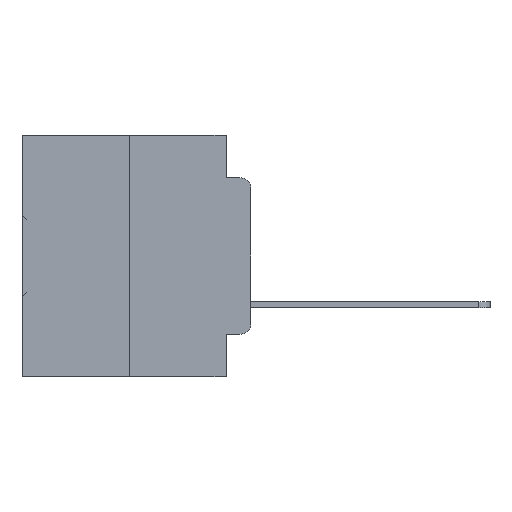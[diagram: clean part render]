
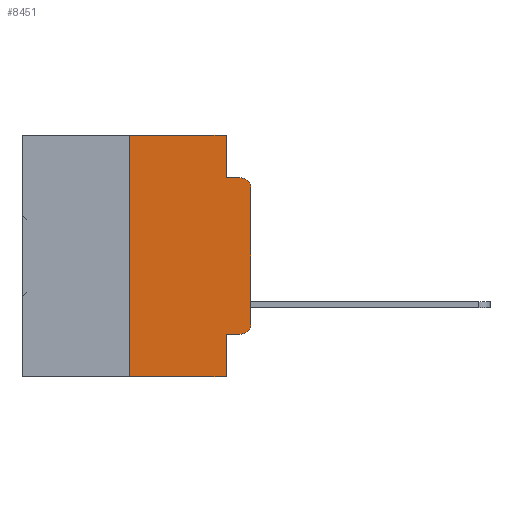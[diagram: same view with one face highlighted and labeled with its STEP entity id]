
A CAD part, left-side view. The second image highlights one B-rep face of the part: STEP entity #8451.
In plain terms, the highlighted planar face has unit normal (-1, 0, 0).
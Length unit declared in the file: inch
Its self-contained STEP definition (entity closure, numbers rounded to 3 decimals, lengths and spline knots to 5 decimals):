
#79 = EDGE_CURVE ( 'NONE', #17918, #13005, #28951, .T. ) ;
#101 = CARTESIAN_POINT ( 'NONE',  ( 0., 0.473, -0.5 ) ) ;
#487 = EDGE_CURVE ( 'NONE', #1792, #5767, #3883, .T. ) ;
#1195 = CARTESIAN_POINT ( 'NONE',  ( 0., 0.051, -0.4115 ) ) ;
#1426 = CIRCLE ( 'NONE', #29211, 0.02 ) ;
#1541 = VERTEX_POINT ( 'NONE', #7631 ) ;
#1792 = VERTEX_POINT ( 'NONE', #15027 ) ;
#2747 = EDGE_LOOP ( 'NONE', ( #7421, #23309, #15810, #28493, #32757, #30654, #3404, #32792, #27252, #3438 ) ) ;
#3170 = PLANE ( 'NONE',  #5697 ) ;
#3185 = EDGE_CURVE ( 'NONE', #1541, #13005, #27560, .T. ) ;
#3294 = DIRECTION ( 'NONE',  ( 0., 0., -1. ) ) ;
#3404 = ORIENTED_EDGE ( 'NONE', *, *, #3185, .T. ) ;
#3438 = ORIENTED_EDGE ( 'NONE', *, *, #20237, .T. ) ;
#3822 = VECTOR ( 'NONE', #32529, 39.37008 ) ;
#3883 = LINE ( 'NONE', #28431, #18070 ) ;
#4495 = CARTESIAN_POINT ( 'NONE',  ( 0., 0.051, 0. ) ) ;
#4998 = CARTESIAN_POINT ( 'NONE',  ( 0., 0., -0.1085 ) ) ;
#5225 = EDGE_CURVE ( 'NONE', #13765, #7297, #27836, .T. ) ;
#5697 = AXIS2_PLACEMENT_3D ( 'NONE', #14611, #20266, #3294 ) ;
#5767 = VERTEX_POINT ( 'NONE', #17756 ) ;
#5954 = DIRECTION ( 'NONE',  ( 0., -1., 0. ) ) ;
#7297 = VERTEX_POINT ( 'NONE', #11140 ) ;
#7421 = ORIENTED_EDGE ( 'NONE', *, *, #27356, .T. ) ;
#7631 = CARTESIAN_POINT ( 'NONE',  ( 0., 0.25, -0.5 ) ) ;
#8050 = LINE ( 'NONE', #35789, #15549 ) ;
#8303 = DIRECTION ( 'NONE',  ( 0., 0., 1. ) ) ;
#8451 = ADVANCED_FACE ( 'NONE', ( #18444 ), #3170, .F. ) ;
#9297 = DIRECTION ( 'NONE',  ( 0., -1., 0. ) ) ;
#11140 = CARTESIAN_POINT ( 'NONE',  ( 0., 0.02, -0.0885 ) ) ;
#11480 = LINE ( 'NONE', #25296, #18086 ) ;
#12324 = VECTOR ( 'NONE', #32002, 39.37008 ) ;
#12492 = DIRECTION ( 'NONE',  ( -1., 0., 0. ) ) ;
#13005 = VERTEX_POINT ( 'NONE', #32638 ) ;
#13181 = LINE ( 'NONE', #4495, #3822 ) ;
#13234 = CARTESIAN_POINT ( 'NONE',  ( 0., 0.02, -0.3915 ) ) ;
#13443 = AXIS2_PLACEMENT_3D ( 'NONE', #29235, #12492, #31969 ) ;
#13765 = VERTEX_POINT ( 'NONE', #4998 ) ;
#14611 = CARTESIAN_POINT ( 'NONE',  ( 0., 0.473, 0. ) ) ;
#15027 = CARTESIAN_POINT ( 'NONE',  ( 0., 0.25, 0. ) ) ;
#15381 = CARTESIAN_POINT ( 'NONE',  ( 0., 0.051, 0. ) ) ;
#15549 = VECTOR ( 'NONE', #35906, 39.37008 ) ;
#15810 = ORIENTED_EDGE ( 'NONE', *, *, #26135, .F. ) ;
#15893 = VECTOR ( 'NONE', #29018, 39.37008 ) ;
#16059 = DIRECTION ( 'NONE',  ( 0., 0., -1. ) ) ;
#17756 = CARTESIAN_POINT ( 'NONE',  ( 0., 0.051, 0. ) ) ;
#17918 = VERTEX_POINT ( 'NONE', #1195 ) ;
#18070 = VECTOR ( 'NONE', #5954, 39.37008 ) ;
#18086 = VECTOR ( 'NONE', #8303, 39.37008 ) ;
#18444 = FACE_OUTER_BOUND ( 'NONE', #2747, .T. ) ;
#19064 = EDGE_CURVE ( 'NONE', #17918, #32541, #35606, .T. ) ;
#19579 = CARTESIAN_POINT ( 'NONE',  ( 0., 0.051, -0.0885 ) ) ;
#20128 = VECTOR ( 'NONE', #30985, 39.37008 ) ;
#20237 = EDGE_CURVE ( 'NONE', #32541, #23037, #1426, .T. ) ;
#20266 = DIRECTION ( 'NONE',  ( 1., 0., 0. ) ) ;
#23037 = VERTEX_POINT ( 'NONE', #29609 ) ;
#23309 = ORIENTED_EDGE ( 'NONE', *, *, #5225, .T. ) ;
#23374 = LINE ( 'NONE', #26274, #15893 ) ;
#24098 = CARTESIAN_POINT ( 'NONE',  ( 0., 0.02, -0.4115 ) ) ;
#25296 = CARTESIAN_POINT ( 'NONE',  ( 0., 0., 0. ) ) ;
#26135 = EDGE_CURVE ( 'NONE', #32149, #7297, #8050, .T. ) ;
#26274 = CARTESIAN_POINT ( 'NONE',  ( 0., 0.25, 0. ) ) ;
#27252 = ORIENTED_EDGE ( 'NONE', *, *, #19064, .T. ) ;
#27356 = EDGE_CURVE ( 'NONE', #23037, #13765, #11480, .T. ) ;
#27521 = VECTOR ( 'NONE', #9297, 39.37008 ) ;
#27560 = LINE ( 'NONE', #101, #20128 ) ;
#27836 = CIRCLE ( 'NONE', #13443, 0.02 ) ;
#28431 = CARTESIAN_POINT ( 'NONE',  ( 0., 0.473, 0. ) ) ;
#28493 = ORIENTED_EDGE ( 'NONE', *, *, #29862, .F. ) ;
#28896 = CARTESIAN_POINT ( 'NONE',  ( 0., 0.051, -0.4115 ) ) ;
#28951 = LINE ( 'NONE', #15381, #12324 ) ;
#29018 = DIRECTION ( 'NONE',  ( 0., 0., 1. ) ) ;
#29211 = AXIS2_PLACEMENT_3D ( 'NONE', #13234, #32680, #16059 ) ;
#29235 = CARTESIAN_POINT ( 'NONE',  ( 0., 0.02, -0.1085 ) ) ;
#29609 = CARTESIAN_POINT ( 'NONE',  ( 0., 0., -0.3915 ) ) ;
#29862 = EDGE_CURVE ( 'NONE', #5767, #32149, #13181, .T. ) ;
#30654 = ORIENTED_EDGE ( 'NONE', *, *, #32424, .F. ) ;
#30985 = DIRECTION ( 'NONE',  ( 0., -1., 0. ) ) ;
#31969 = DIRECTION ( 'NONE',  ( 0., 0., -1. ) ) ;
#32002 = DIRECTION ( 'NONE',  ( 0., 0., -1. ) ) ;
#32149 = VERTEX_POINT ( 'NONE', #19579 ) ;
#32424 = EDGE_CURVE ( 'NONE', #1541, #1792, #23374, .T. ) ;
#32529 = DIRECTION ( 'NONE',  ( 0., 0., -1. ) ) ;
#32541 = VERTEX_POINT ( 'NONE', #24098 ) ;
#32638 = CARTESIAN_POINT ( 'NONE',  ( 0., 0.051, -0.5 ) ) ;
#32680 = DIRECTION ( 'NONE',  ( -1., 0., 0. ) ) ;
#32757 = ORIENTED_EDGE ( 'NONE', *, *, #487, .F. ) ;
#32792 = ORIENTED_EDGE ( 'NONE', *, *, #79, .F. ) ;
#35606 = LINE ( 'NONE', #28896, #27521 ) ;
#35789 = CARTESIAN_POINT ( 'NONE',  ( 0., 0.051, -0.0885 ) ) ;
#35906 = DIRECTION ( 'NONE',  ( 0., -1., 0. ) ) ;
